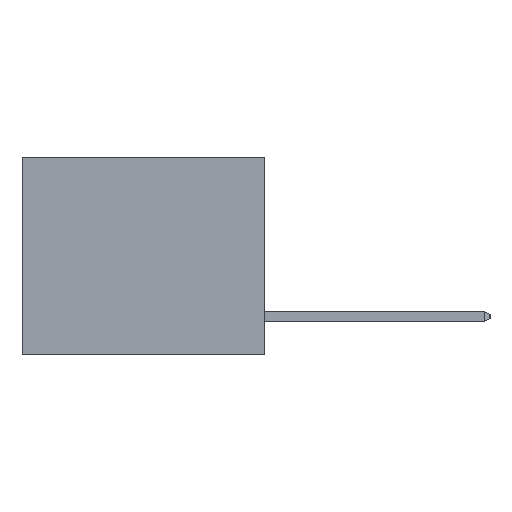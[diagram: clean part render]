
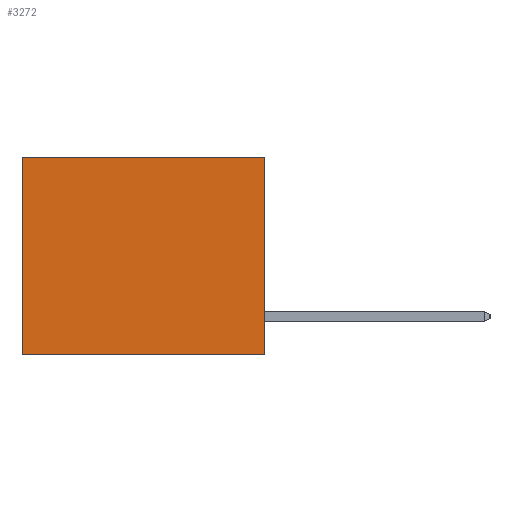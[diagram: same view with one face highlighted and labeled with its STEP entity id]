
A CAD part, left-side view. The second image highlights one B-rep face of the part: STEP entity #3272.
In plain terms, the highlighted planar face has unit normal (-1, 0, 0).
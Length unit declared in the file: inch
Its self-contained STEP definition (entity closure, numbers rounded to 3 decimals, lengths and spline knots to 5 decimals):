
#127 = FACE_OUTER_BOUND ( 'NONE', #12637, .T. ) ;
#445 = CARTESIAN_POINT ( 'NONE',  ( 0.3165, 0., -0.49 ) ) ;
#2006 = DIRECTION ( 'NONE',  ( 0., 0., -1. ) ) ;
#2134 = LINE ( 'NONE', #445, #20061 ) ;
#2152 = DIRECTION ( 'NONE',  ( 0., 1., 0. ) ) ;
#3272 = ADVANCED_FACE ( 'NONE', ( #127 ), #6744, .F. ) ;
#3320 = LINE ( 'NONE', #5374, #3865 ) ;
#3865 = VECTOR ( 'NONE', #2006, 39.37008 ) ;
#4130 = CARTESIAN_POINT ( 'NONE',  ( 0.3165, 0., 0. ) ) ;
#4281 = VERTEX_POINT ( 'NONE', #21568 ) ;
#5374 = CARTESIAN_POINT ( 'NONE',  ( 0.3165, 0., -0.49 ) ) ;
#5528 = ORIENTED_EDGE ( 'NONE', *, *, #18792, .T. ) ;
#6744 = PLANE ( 'NONE',  #22530 ) ;
#8247 = ORIENTED_EDGE ( 'NONE', *, *, #22181, .F. ) ;
#9148 = CARTESIAN_POINT ( 'NONE',  ( 0.3165, 0.6, -0.49 ) ) ;
#10109 = ORIENTED_EDGE ( 'NONE', *, *, #18820, .T. ) ;
#10238 = CARTESIAN_POINT ( 'NONE',  ( 0.3165, 0., -0.49 ) ) ;
#10404 = VECTOR ( 'NONE', #16045, 39.37008 ) ;
#12235 = CARTESIAN_POINT ( 'NONE',  ( 0.3165, 0.6, -0.49 ) ) ;
#12637 = EDGE_LOOP ( 'NONE', ( #5528, #8247, #22385, #10109 ) ) ;
#12880 = VECTOR ( 'NONE', #16116, 39.37008 ) ;
#13763 = DIRECTION ( 'NONE',  ( 0., 0., -1. ) ) ;
#15569 = LINE ( 'NONE', #4130, #10404 ) ;
#16045 = DIRECTION ( 'NONE',  ( 0., 1., 0. ) ) ;
#16070 = CARTESIAN_POINT ( 'NONE',  ( 0.3165, 0., -0.49 ) ) ;
#16110 = VERTEX_POINT ( 'NONE', #16070 ) ;
#16116 = DIRECTION ( 'NONE',  ( 0., 0., -1. ) ) ;
#18543 = LINE ( 'NONE', #9148, #12880 ) ;
#18792 = EDGE_CURVE ( 'NONE', #22150, #20784, #18543, .T. ) ;
#18820 = EDGE_CURVE ( 'NONE', #4281, #22150, #15569, .T. ) ;
#19145 = EDGE_CURVE ( 'NONE', #4281, #16110, #3320, .T. ) ;
#20061 = VECTOR ( 'NONE', #2152, 39.37008 ) ;
#20784 = VERTEX_POINT ( 'NONE', #12235 ) ;
#21278 = CARTESIAN_POINT ( 'NONE',  ( 0.3165, 0.6, 0. ) ) ;
#21568 = CARTESIAN_POINT ( 'NONE',  ( 0.3165, 0., 0. ) ) ;
#22150 = VERTEX_POINT ( 'NONE', #21278 ) ;
#22181 = EDGE_CURVE ( 'NONE', #16110, #20784, #2134, .T. ) ;
#22220 = DIRECTION ( 'NONE',  ( 1., 0., 0. ) ) ;
#22385 = ORIENTED_EDGE ( 'NONE', *, *, #19145, .F. ) ;
#22530 = AXIS2_PLACEMENT_3D ( 'NONE', #10238, #22220, #13763 ) ;
